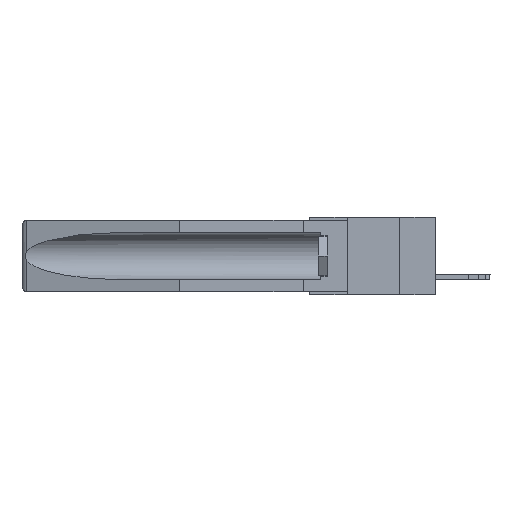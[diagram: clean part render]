
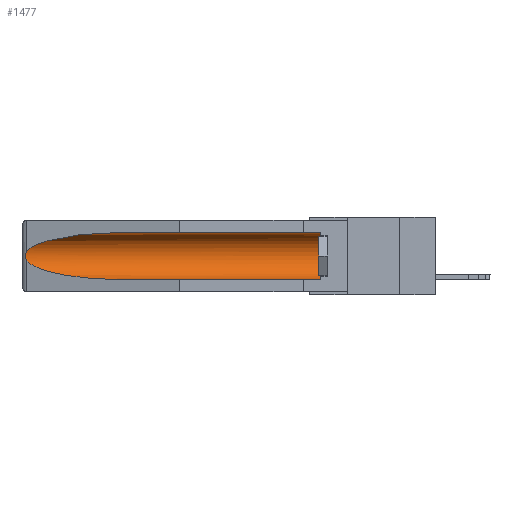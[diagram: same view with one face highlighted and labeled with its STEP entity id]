
A CAD part, left-side view. The second image highlights one B-rep face of the part: STEP entity #1477.
In plain terms, the highlighted cylindrical face has radius 2.857 mm (diameter 5.715 mm), a partial arc.
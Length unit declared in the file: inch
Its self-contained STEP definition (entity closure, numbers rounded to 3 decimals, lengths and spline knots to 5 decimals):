
#283 = CARTESIAN_POINT ( 'NONE',  ( 0.155, -0.30754, -0.059 ) ) ;
#609 = CARTESIAN_POINT ( 'NONE',  ( 0.25451, 1.48313, -0.24835 ) ) ;
#636 = VERTEX_POINT ( 'NONE', #1990 ) ;
#1344 = EDGE_CURVE ( 'NONE', #12810, #636, #9659, .T. ) ;
#1435 = CARTESIAN_POINT ( 'NONE',  ( 0.2675, 1.53308, -0.16763 ) ) ;
#1456 = EDGE_CURVE ( 'NONE', #12810, #13067, #16208, .T. ) ;
#1477 = ADVANCED_FACE ( 'NONE', ( #3417 ), #2645, .F. ) ;
#1990 = CARTESIAN_POINT ( 'NONE',  ( 0.155, 0.126, -0.059 ) ) ;
#2142 = EDGE_CURVE ( 'NONE', #11492, #15771, #13524, .T. ) ;
#2573 =( BOUNDED_CURVE ( )  B_SPLINE_CURVE ( 3, ( #13286, #15988, #5733, #5783 ),
 .UNSPECIFIED., .F., .F. ) 
 B_SPLINE_CURVE_WITH_KNOTS ( ( 4, 4 ),
 ( 4.71239, 6.08839 ),
 .UNSPECIFIED. ) 
 CURVE ( )  GEOMETRIC_REPRESENTATION_ITEM ( )  RATIONAL_B_SPLINE_CURVE ( ( 1., 0.848, 0.848, 1. ) ) 
 REPRESENTATION_ITEM ( '' )  );
#2645 = CYLINDRICAL_SURFACE ( 'NONE', #10248, 0.1125 ) ;
#2764 = CARTESIAN_POINT ( 'NONE',  ( 0.26537, 1.52718, -0.19328 ) ) ;
#3045 = ORIENTED_EDGE ( 'NONE', *, *, #1456, .F. ) ;
#3253 = EDGE_LOOP ( 'NONE', ( #6739, #8317, #14217, #3045, #14391, #10278 ) ) ;
#3345 = CARTESIAN_POINT ( 'NONE',  ( 0.155, -0.30754, -0.1715 ) ) ;
#3417 = FACE_OUTER_BOUND ( 'NONE', #3253, .T. ) ;
#3695 = CARTESIAN_POINT ( 'NONE',  ( 0.26537, 1.52718, -0.14972 ) ) ;
#3876 =( BOUNDED_CURVE ( )  B_SPLINE_CURVE ( 3, ( #4950, #609, #15828, #9664 ),
 .UNSPECIFIED., .F., .F. ) 
 B_SPLINE_CURVE_WITH_KNOTS ( ( 4, 4 ),
 ( 0.1948, 1.5708 ),
 .UNSPECIFIED. ) 
 CURVE ( )  GEOMETRIC_REPRESENTATION_ITEM ( )  RATIONAL_B_SPLINE_CURVE ( ( 1., 0.848, 0.848, 1. ) ) 
 REPRESENTATION_ITEM ( '' )  );
#4282 = EDGE_CURVE ( 'NONE', #15771, #13067, #3876, .T. ) ;
#4558 = CARTESIAN_POINT ( 'NONE',  ( 0.155, 0.126, -0.284 ) ) ;
#4630 = DIRECTION ( 'NONE',  ( 0., 1., 0. ) ) ;
#4818 = CARTESIAN_POINT ( 'NONE',  ( 0.26537, 1.52718, -0.14972 ) ) ;
#4950 = CARTESIAN_POINT ( 'NONE',  ( 0.26537, 1.52718, -0.19328 ) ) ;
#5309 = EDGE_CURVE ( 'NONE', #14927, #11492, #2573, .T. ) ;
#5733 = CARTESIAN_POINT ( 'NONE',  ( 0.25451, 1.48313, -0.09465 ) ) ;
#5783 = CARTESIAN_POINT ( 'NONE',  ( 0.26537, 1.52718, -0.14972 ) ) ;
#6739 = ORIENTED_EDGE ( 'NONE', *, *, #5309, .T. ) ;
#7119 = DIRECTION ( 'NONE',  ( 0., 0., 1. ) ) ;
#7654 = CARTESIAN_POINT ( 'NONE',  ( 0.26654, 1.53092, -0.15636 ) ) ;
#8317 = ORIENTED_EDGE ( 'NONE', *, *, #2142, .T. ) ;
#8390 = DIRECTION ( 'NONE',  ( 0., 1., 0. ) ) ;
#8700 = LINE ( 'NONE', #283, #11290 ) ;
#8701 = CARTESIAN_POINT ( 'NONE',  ( 0.26597, 1.52961, -0.15275 ) ) ;
#8858 = CARTESIAN_POINT ( 'NONE',  ( 0.155, 1.07973, -0.059 ) ) ;
#9058 = CARTESIAN_POINT ( 'NONE',  ( 0.2675, 1.53308, -0.17534 ) ) ;
#9659 = CIRCLE ( 'NONE', #16187, 0.1125 ) ;
#9664 = CARTESIAN_POINT ( 'NONE',  ( 0.155, 1.07973, -0.284 ) ) ;
#10248 = AXIS2_PLACEMENT_3D ( 'NONE', #3345, #4630, #7119 ) ;
#10278 = ORIENTED_EDGE ( 'NONE', *, *, #12531, .T. ) ;
#11290 = VECTOR ( 'NONE', #11787, 39.37008 ) ;
#11492 = VERTEX_POINT ( 'NONE', #4818 ) ;
#11605 = CARTESIAN_POINT ( 'NONE',  ( 0.26597, 1.5296, -0.19026 ) ) ;
#11787 = DIRECTION ( 'NONE',  ( 0., 1., 0. ) ) ;
#12531 = EDGE_CURVE ( 'NONE', #636, #14927, #8700, .T. ) ;
#12777 = CARTESIAN_POINT ( 'NONE',  ( 0.2673, 1.5327, -0.16383 ) ) ;
#12810 = VERTEX_POINT ( 'NONE', #4558 ) ;
#12836 = CARTESIAN_POINT ( 'NONE',  ( 0.26655, 1.53094, -0.18657 ) ) ;
#12898 = CARTESIAN_POINT ( 'NONE',  ( 0.2673, 1.53269, -0.17917 ) ) ;
#13067 = VERTEX_POINT ( 'NONE', #15777 ) ;
#13286 = CARTESIAN_POINT ( 'NONE',  ( 0.155, 1.07973, -0.059 ) ) ;
#13524 = B_SPLINE_CURVE_WITH_KNOTS ( 'NONE', 3,
 ( #3695, #8701, #7654, #12777, #1435, #9058, #12898, #12836, #11605, #2764 ),
 .UNSPECIFIED., .F., .F.,
 ( 4, 2, 2, 2, 4 ),
 ( 0., 0.00029, 0.00058, 0.00087, 0.00117 ),
 .UNSPECIFIED. ) ;
#13837 = DIRECTION ( 'NONE',  ( 0., -1., 0. ) ) ;
#14217 = ORIENTED_EDGE ( 'NONE', *, *, #4282, .T. ) ;
#14391 = ORIENTED_EDGE ( 'NONE', *, *, #1344, .T. ) ;
#14758 = CARTESIAN_POINT ( 'NONE',  ( 0.155, 0.126, -0.1715 ) ) ;
#14910 = CARTESIAN_POINT ( 'NONE',  ( 0.26537, 1.52718, -0.19328 ) ) ;
#14927 = VERTEX_POINT ( 'NONE', #8858 ) ;
#14969 = DIRECTION ( 'NONE',  ( 0., 0., 1. ) ) ;
#15771 = VERTEX_POINT ( 'NONE', #14910 ) ;
#15777 = CARTESIAN_POINT ( 'NONE',  ( 0.155, 1.07973, -0.284 ) ) ;
#15828 = CARTESIAN_POINT ( 'NONE',  ( 0.21114, 1.30732, -0.284 ) ) ;
#15988 = CARTESIAN_POINT ( 'NONE',  ( 0.21114, 1.30732, -0.059 ) ) ;
#16023 = CARTESIAN_POINT ( 'NONE',  ( 0.155, -0.30754, -0.284 ) ) ;
#16187 = AXIS2_PLACEMENT_3D ( 'NONE', #14758, #13837, #14969 ) ;
#16208 = LINE ( 'NONE', #16023, #16444 ) ;
#16444 = VECTOR ( 'NONE', #8390, 39.37008 ) ;
